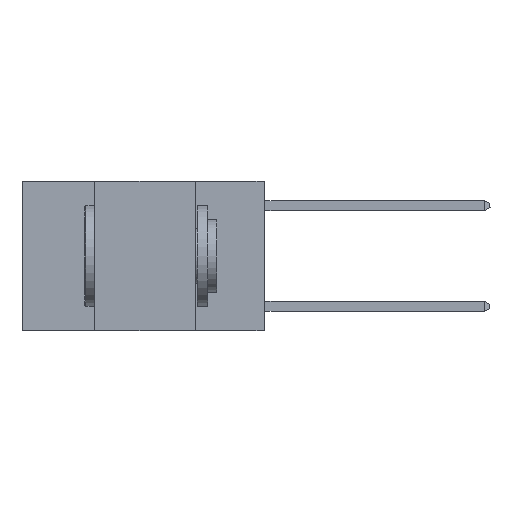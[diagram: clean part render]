
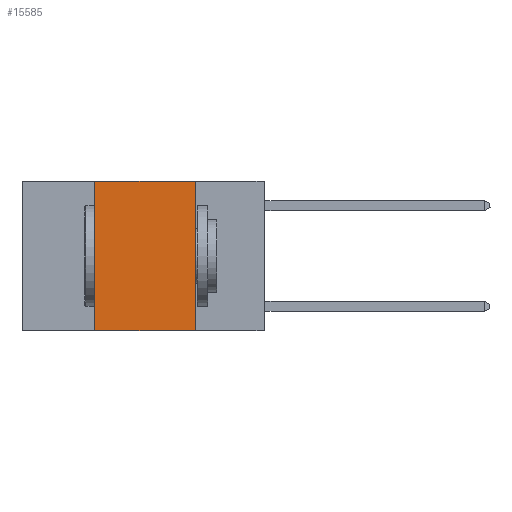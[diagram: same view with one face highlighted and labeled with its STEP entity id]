
A CAD part, left-side view. The second image highlights one B-rep face of the part: STEP entity #15585.
In plain terms, the highlighted planar face has unit normal (-1, 0, 0).
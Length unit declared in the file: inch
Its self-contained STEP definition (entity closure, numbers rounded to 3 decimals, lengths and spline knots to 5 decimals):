
#107 = ORIENTED_EDGE ( 'NONE', *, *, #2529, .F. ) ;
#957 = DIRECTION ( 'NONE',  ( 0., 0., -1. ) ) ;
#1480 = LINE ( 'NONE', #9145, #7982 ) ;
#2457 = LINE ( 'NONE', #16822, #9350 ) ;
#2529 = EDGE_CURVE ( 'NONE', #12628, #3793, #1480, .T. ) ;
#3206 = ORIENTED_EDGE ( 'NONE', *, *, #13933, .F. ) ;
#3590 = FACE_OUTER_BOUND ( 'NONE', #13384, .T. ) ;
#3793 = VERTEX_POINT ( 'NONE', #6820 ) ;
#4058 = DIRECTION ( 'NONE',  ( 0., -1., 0. ) ) ;
#4442 = CARTESIAN_POINT ( 'NONE',  ( 0., 0.17, 0. ) ) ;
#4530 = DIRECTION ( 'NONE',  ( 1., 0., 0. ) ) ;
#6627 = ORIENTED_EDGE ( 'NONE', *, *, #13621, .F. ) ;
#6820 = CARTESIAN_POINT ( 'NONE',  ( 0., 0.42, 0. ) ) ;
#6852 = VERTEX_POINT ( 'NONE', #7792 ) ;
#7204 = CARTESIAN_POINT ( 'NONE',  ( 0., 0.42, -0.37 ) ) ;
#7792 = CARTESIAN_POINT ( 'NONE',  ( 0., 0.17, -0.37 ) ) ;
#7982 = VECTOR ( 'NONE', #9044, 39.37008 ) ;
#8121 = LINE ( 'NONE', #10073, #15027 ) ;
#8223 = AXIS2_PLACEMENT_3D ( 'NONE', #16166, #4530, #13637 ) ;
#8401 = PLANE ( 'NONE',  #8223 ) ;
#9044 = DIRECTION ( 'NONE',  ( 0., 0., 1. ) ) ;
#9145 = CARTESIAN_POINT ( 'NONE',  ( 0., 0.42, 0. ) ) ;
#9350 = VECTOR ( 'NONE', #10395, 39.37008 ) ;
#9983 = LINE ( 'NONE', #14556, #13021 ) ;
#10073 = CARTESIAN_POINT ( 'NONE',  ( 0., 0.17, 0. ) ) ;
#10395 = DIRECTION ( 'NONE',  ( 0., -1., 0. ) ) ;
#10540 = ORIENTED_EDGE ( 'NONE', *, *, #13441, .T. ) ;
#12628 = VERTEX_POINT ( 'NONE', #7204 ) ;
#13021 = VECTOR ( 'NONE', #4058, 39.37008 ) ;
#13384 = EDGE_LOOP ( 'NONE', ( #3206, #6627, #107, #10540 ) ) ;
#13441 = EDGE_CURVE ( 'NONE', #12628, #6852, #2457, .T. ) ;
#13621 = EDGE_CURVE ( 'NONE', #3793, #13732, #9983, .T. ) ;
#13637 = DIRECTION ( 'NONE',  ( 0., 0., -1. ) ) ;
#13732 = VERTEX_POINT ( 'NONE', #4442 ) ;
#13933 = EDGE_CURVE ( 'NONE', #13732, #6852, #8121, .T. ) ;
#14556 = CARTESIAN_POINT ( 'NONE',  ( 0., 0.6, 0. ) ) ;
#15027 = VECTOR ( 'NONE', #957, 39.37008 ) ;
#15585 = ADVANCED_FACE ( 'NONE', ( #3590 ), #8401, .F. ) ;
#16166 = CARTESIAN_POINT ( 'NONE',  ( 0., 0.6, 0. ) ) ;
#16822 = CARTESIAN_POINT ( 'NONE',  ( 0., 0.6, -0.37 ) ) ;
